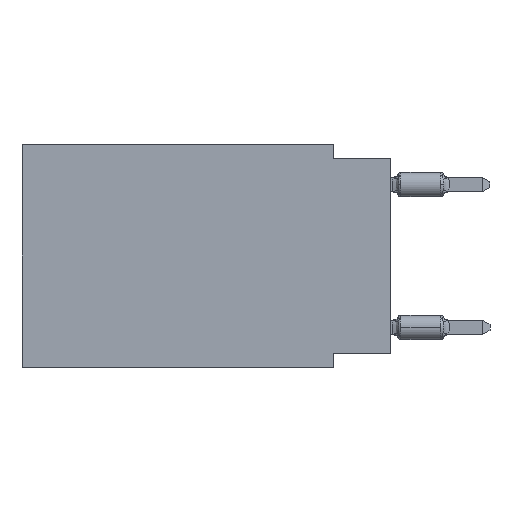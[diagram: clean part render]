
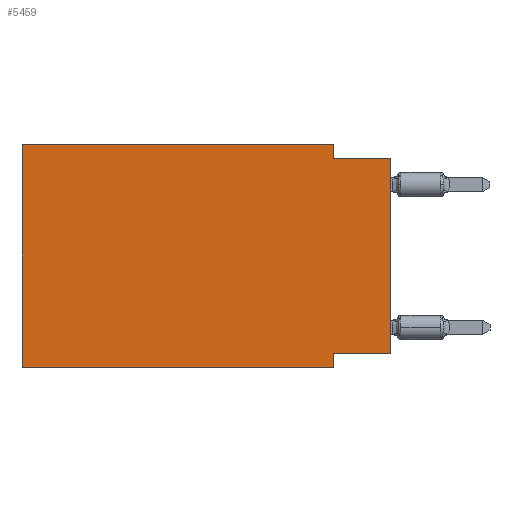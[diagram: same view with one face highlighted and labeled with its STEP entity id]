
A CAD part, left-side view. The second image highlights one B-rep face of the part: STEP entity #5459.
In plain terms, the highlighted planar face has unit normal (-1, 0, 0).
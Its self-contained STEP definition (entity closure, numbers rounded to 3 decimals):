
#25 = CARTESIAN_POINT ( 'NONE',  ( 0., 16.383, -9.906 ) ) ;
#278 = CARTESIAN_POINT ( 'NONE',  ( 0., 16.383, 0. ) ) ;
#355 = CARTESIAN_POINT ( 'NONE',  ( 0., 0., -0.635 ) ) ;
#543 = LINE ( 'NONE', #355, #6292 ) ;
#751 = CARTESIAN_POINT ( 'NONE',  ( 0., 16.383, 0. ) ) ;
#838 = ORIENTED_EDGE ( 'NONE', *, *, #8886, .T. ) ;
#1423 = VERTEX_POINT ( 'NONE', #16429 ) ;
#1647 = DIRECTION ( 'NONE',  ( 0., 0., 1. ) ) ;
#1944 = CARTESIAN_POINT ( 'NONE',  ( 0., 0., -9.271 ) ) ;
#2272 = DIRECTION ( 'NONE',  ( 0., 0., 1. ) ) ;
#2687 = CARTESIAN_POINT ( 'NONE',  ( 0., 2.54, -9.906 ) ) ;
#3229 = ORIENTED_EDGE ( 'NONE', *, *, #10395, .F. ) ;
#3555 = DIRECTION ( 'NONE',  ( 0., -1., 0. ) ) ;
#3909 = VERTEX_POINT ( 'NONE', #13704 ) ;
#4411 = VECTOR ( 'NONE', #2272, 1000. ) ;
#4554 = CARTESIAN_POINT ( 'NONE',  ( 0., 0., 0. ) ) ;
#4640 = VERTEX_POINT ( 'NONE', #1944 ) ;
#4768 = DIRECTION ( 'NONE',  ( 1., 0., 0. ) ) ;
#4876 = VERTEX_POINT ( 'NONE', #18175 ) ;
#5172 = VECTOR ( 'NONE', #11029, 1000. ) ;
#5393 = DIRECTION ( 'NONE',  ( 0., -1., 0. ) ) ;
#5445 = EDGE_LOOP ( 'NONE', ( #11208, #17458, #9879, #15003, #3229, #838, #16350, #8080 ) ) ;
#5459 = ADVANCED_FACE ( 'NONE', ( #17370 ), #13124, .F. ) ;
#5679 = VERTEX_POINT ( 'NONE', #17813 ) ;
#5715 = LINE ( 'NONE', #11413, #14517 ) ;
#6168 = EDGE_CURVE ( 'NONE', #4640, #7803, #9705, .T. ) ;
#6241 = EDGE_CURVE ( 'NONE', #7803, #5679, #9982, .T. ) ;
#6263 = DIRECTION ( 'NONE',  ( 0., -1., 0. ) ) ;
#6292 = VECTOR ( 'NONE', #6263, 1000. ) ;
#6365 = AXIS2_PLACEMENT_3D ( 'NONE', #278, #4768, #13307 ) ;
#7603 = EDGE_CURVE ( 'NONE', #4640, #3909, #14527, .T. ) ;
#7803 = VERTEX_POINT ( 'NONE', #11466 ) ;
#8080 = ORIENTED_EDGE ( 'NONE', *, *, #6168, .F. ) ;
#8318 = CARTESIAN_POINT ( 'NONE',  ( 0., 0., -9.271 ) ) ;
#8758 = VECTOR ( 'NONE', #5393, 1000. ) ;
#8886 = EDGE_CURVE ( 'NONE', #4876, #5679, #15526, .T. ) ;
#9434 = EDGE_CURVE ( 'NONE', #11214, #3909, #543, .T. ) ;
#9705 = LINE ( 'NONE', #8318, #14192 ) ;
#9879 = ORIENTED_EDGE ( 'NONE', *, *, #14881, .F. ) ;
#9982 = LINE ( 'NONE', #2687, #5172 ) ;
#10395 = EDGE_CURVE ( 'NONE', #4876, #16805, #15225, .T. ) ;
#11029 = DIRECTION ( 'NONE',  ( 0., 0., -1. ) ) ;
#11208 = ORIENTED_EDGE ( 'NONE', *, *, #7603, .T. ) ;
#11214 = VERTEX_POINT ( 'NONE', #14330 ) ;
#11413 = CARTESIAN_POINT ( 'NONE',  ( 0., 2.54, 0. ) ) ;
#11466 = CARTESIAN_POINT ( 'NONE',  ( 0., 2.54, -9.271 ) ) ;
#11541 = CARTESIAN_POINT ( 'NONE',  ( 0., 16.383, 0. ) ) ;
#11687 = DIRECTION ( 'NONE',  ( 0., 0., -1. ) ) ;
#11950 = EDGE_CURVE ( 'NONE', #16805, #1423, #16422, .T. ) ;
#12384 = CARTESIAN_POINT ( 'NONE',  ( 0., 16.383, 0. ) ) ;
#13124 = PLANE ( 'NONE',  #6365 ) ;
#13307 = DIRECTION ( 'NONE',  ( 0., 0., -1. ) ) ;
#13704 = CARTESIAN_POINT ( 'NONE',  ( 0., 0., -0.635 ) ) ;
#14049 = DIRECTION ( 'NONE',  ( 0., 1., 0. ) ) ;
#14192 = VECTOR ( 'NONE', #14049, 1000. ) ;
#14330 = CARTESIAN_POINT ( 'NONE',  ( 0., 2.54, -0.635 ) ) ;
#14517 = VECTOR ( 'NONE', #11687, 1000. ) ;
#14527 = LINE ( 'NONE', #4554, #18034 ) ;
#14881 = EDGE_CURVE ( 'NONE', #1423, #11214, #5715, .T. ) ;
#15003 = ORIENTED_EDGE ( 'NONE', *, *, #11950, .F. ) ;
#15225 = LINE ( 'NONE', #12384, #4411 ) ;
#15526 = LINE ( 'NONE', #25, #8758 ) ;
#16350 = ORIENTED_EDGE ( 'NONE', *, *, #6241, .F. ) ;
#16422 = LINE ( 'NONE', #751, #16750 ) ;
#16429 = CARTESIAN_POINT ( 'NONE',  ( 0., 2.54, 0. ) ) ;
#16750 = VECTOR ( 'NONE', #3555, 1000. ) ;
#16805 = VERTEX_POINT ( 'NONE', #11541 ) ;
#17370 = FACE_OUTER_BOUND ( 'NONE', #5445, .T. ) ;
#17458 = ORIENTED_EDGE ( 'NONE', *, *, #9434, .F. ) ;
#17813 = CARTESIAN_POINT ( 'NONE',  ( 0., 2.54, -9.906 ) ) ;
#18034 = VECTOR ( 'NONE', #1647, 1000. ) ;
#18175 = CARTESIAN_POINT ( 'NONE',  ( 0., 16.383, -9.906 ) ) ;
